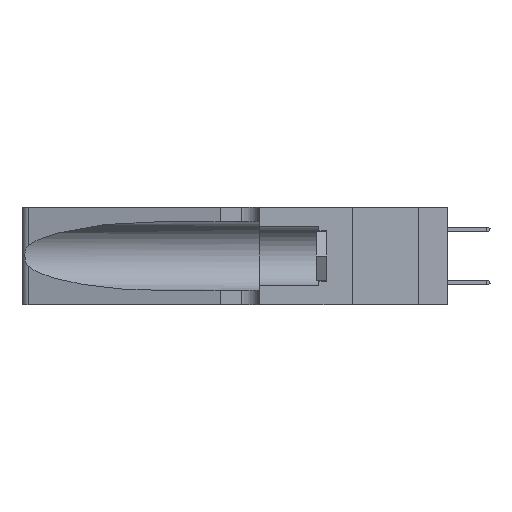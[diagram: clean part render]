
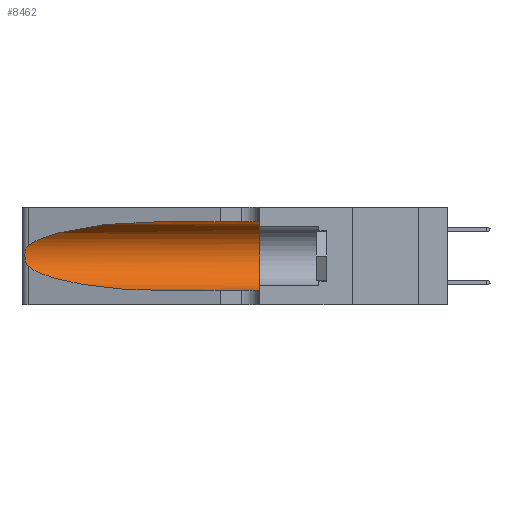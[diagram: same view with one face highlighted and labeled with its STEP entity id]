
A CAD part, left-side view. The second image highlights one B-rep face of the part: STEP entity #8462.
In plain terms, the highlighted cylindrical face has radius 3.308 mm (diameter 6.617 mm), a partial arc.
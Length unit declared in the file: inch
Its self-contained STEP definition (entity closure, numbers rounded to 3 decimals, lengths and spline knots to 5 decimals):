
#17 = EDGE_CURVE ( 'NONE', #8812, #5619, #6114, .T. ) ;
#32 = CARTESIAN_POINT ( 'NONE',  ( 0.25555, 1.22993, 0.14849 ) ) ;
#1219 = ORIENTED_EDGE ( 'NONE', *, *, #14206, .T. ) ;
#1509 = CARTESIAN_POINT ( 'NONE',  ( 0.25487, 1.22718, 0.22369 ) ) ;
#1870 = B_SPLINE_CURVE_WITH_KNOTS ( 'NONE', 3,
 ( #8646, #10775, #17141, #4388, #19278, #6592, #21378, #8741, #23460, #10874, #25539, #12975, #32, #15109 ),
 .UNSPECIFIED., .F., .F.,
 ( 4, 2, 2, 2, 2, 2, 4 ),
 ( 0., 0.00027, 0.00053, 0.00107, 0.0016, 0.00187, 0.00214 ),
 .UNSPECIFIED. ) ;
#2172 = FACE_OUTER_BOUND ( 'NONE', #9731, .T. ) ;
#3289 = VERTEX_POINT ( 'NONE', #6170 ) ;
#4388 = CARTESIAN_POINT ( 'NONE',  ( 0.25787, 1.23484, 0.2124 ) ) ;
#4996 = CARTESIAN_POINT ( 'NONE',  ( 0.25487, 1.22718, 0.14631 ) ) ;
#5226 = CARTESIAN_POINT ( 'NONE',  ( 0.1305, 0.72297, 0.05475 ) ) ;
#5433 = ORIENTED_EDGE ( 'NONE', *, *, #27164, .T. ) ;
#5501 = EDGE_CURVE ( 'NONE', #9207, #23455, #18853, .T. ) ;
#5619 = VERTEX_POINT ( 'NONE', #19487 ) ;
#5722 = AXIS2_PLACEMENT_3D ( 'NONE', #21940, #9316, #24040 ) ;
#5958 = VECTOR ( 'NONE', #11796, 39.37008 ) ;
#6114 =( BOUNDED_CURVE ( )  B_SPLINE_CURVE ( 3, ( #16597, #17229, #24713, #1509 ),
 .UNSPECIFIED., .F., .T. ) 
 B_SPLINE_CURVE_WITH_KNOTS ( ( 4, 4 ),
 ( 1.5708, 2.84003 ),
 .UNSPECIFIED. ) 
 CURVE ( )  GEOMETRIC_REPRESENTATION_ITEM ( )  RATIONAL_B_SPLINE_CURVE ( ( 1., 0.87, 0.87, 1. ) ) 
 REPRESENTATION_ITEM ( '' )  );
#6170 = CARTESIAN_POINT ( 'NONE',  ( 0.1305, 0.35, 0.31525 ) ) ;
#6348 = CARTESIAN_POINT ( 'NONE',  ( 0.25487, 1.22718, 0.14631 ) ) ;
#6394 = VECTOR ( 'NONE', #26778, 39.37008 ) ;
#6592 = CARTESIAN_POINT ( 'NONE',  ( 0.26018, 1.23835, 0.19895 ) ) ;
#6639 = CYLINDRICAL_SURFACE ( 'NONE', #16690, 0.13025 ) ;
#6921 = ORIENTED_EDGE ( 'NONE', *, *, #5501, .T. ) ;
#7614 = DIRECTION ( 'NONE',  ( 0., -1., 0. ) ) ;
#7970 = LINE ( 'NONE', #9660, #5958 ) ;
#8048 = ORIENTED_EDGE ( 'NONE', *, *, #17980, .F. ) ;
#8462 = ADVANCED_FACE ( 'NONE', ( #2172 ), #6639, .F. ) ;
#8500 = CARTESIAN_POINT ( 'NONE',  ( 0.1305, 0.72297, 0.05475 ) ) ;
#8646 = CARTESIAN_POINT ( 'NONE',  ( 0.25487, 1.22718, 0.22369 ) ) ;
#8741 = CARTESIAN_POINT ( 'NONE',  ( 0.26075, 1.23896, 0.178 ) ) ;
#8812 = VERTEX_POINT ( 'NONE', #26866 ) ;
#9207 = VERTEX_POINT ( 'NONE', #4996 ) ;
#9316 = DIRECTION ( 'NONE',  ( 0., 1., 0. ) ) ;
#9354 = CARTESIAN_POINT ( 'NONE',  ( 0.1305, 0.35, 0.05475 ) ) ;
#9660 = CARTESIAN_POINT ( 'NONE',  ( 0.1305, 1.61858, 0.05475 ) ) ;
#9731 = EDGE_LOOP ( 'NONE', ( #12218, #5433, #6921, #1219, #25384, #8048 ) ) ;
#10504 = VERTEX_POINT ( 'NONE', #9354 ) ;
#10775 = CARTESIAN_POINT ( 'NONE',  ( 0.25555, 1.22994, 0.2215 ) ) ;
#10874 = CARTESIAN_POINT ( 'NONE',  ( 0.25856, 1.23593, 0.16098 ) ) ;
#11130 = EDGE_CURVE ( 'NONE', #3289, #10504, #13754, .T. ) ;
#11786 = DIRECTION ( 'NONE',  ( 0., 0., -1. ) ) ;
#11796 = DIRECTION ( 'NONE',  ( 0., -1., 0. ) ) ;
#12218 = ORIENTED_EDGE ( 'NONE', *, *, #17, .T. ) ;
#12975 = CARTESIAN_POINT ( 'NONE',  ( 0.25639, 1.23186, 0.15144 ) ) ;
#13754 = CIRCLE ( 'NONE', #5722, 0.13025 ) ;
#14206 = EDGE_CURVE ( 'NONE', #23455, #10504, #7970, .T. ) ;
#15109 = CARTESIAN_POINT ( 'NONE',  ( 0.25487, 1.22718, 0.14631 ) ) ;
#16597 = CARTESIAN_POINT ( 'NONE',  ( 0.1305, 0.72297, 0.31525 ) ) ;
#16690 = AXIS2_PLACEMENT_3D ( 'NONE', #22353, #7614, #11786 ) ;
#16906 = CARTESIAN_POINT ( 'NONE',  ( 0.2373, 1.15595, 0.08982 ) ) ;
#17141 = CARTESIAN_POINT ( 'NONE',  ( 0.25639, 1.23184, 0.21858 ) ) ;
#17229 = CARTESIAN_POINT ( 'NONE',  ( 0.18966, 0.96281, 0.31525 ) ) ;
#17980 = EDGE_CURVE ( 'NONE', #8812, #3289, #23224, .T. ) ;
#18853 =( BOUNDED_CURVE ( )  B_SPLINE_CURVE ( 3, ( #6348, #16906, #21138, #8500 ),
 .UNSPECIFIED., .F., .F. ) 
 B_SPLINE_CURVE_WITH_KNOTS ( ( 4, 4 ),
 ( 3.44316, 4.71239 ),
 .UNSPECIFIED. ) 
 CURVE ( )  GEOMETRIC_REPRESENTATION_ITEM ( )  RATIONAL_B_SPLINE_CURVE ( ( 1., 0.87, 0.87, 1. ) ) 
 REPRESENTATION_ITEM ( '' )  );
#19278 = CARTESIAN_POINT ( 'NONE',  ( 0.25854, 1.2359, 0.20912 ) ) ;
#19487 = CARTESIAN_POINT ( 'NONE',  ( 0.25487, 1.22718, 0.22369 ) ) ;
#20513 = CARTESIAN_POINT ( 'NONE',  ( 0.1305, 1.61858, 0.31525 ) ) ;
#21138 = CARTESIAN_POINT ( 'NONE',  ( 0.18966, 0.96281, 0.05475 ) ) ;
#21378 = CARTESIAN_POINT ( 'NONE',  ( 0.26075, 1.23896, 0.19203 ) ) ;
#21940 = CARTESIAN_POINT ( 'NONE',  ( 0.1305, 0.35, 0.185 ) ) ;
#22353 = CARTESIAN_POINT ( 'NONE',  ( 0.1305, 1.61858, 0.185 ) ) ;
#23224 = LINE ( 'NONE', #20513, #6394 ) ;
#23455 = VERTEX_POINT ( 'NONE', #5226 ) ;
#23460 = CARTESIAN_POINT ( 'NONE',  ( 0.26017, 1.23833, 0.17102 ) ) ;
#24040 = DIRECTION ( 'NONE',  ( 0., 0., 1. ) ) ;
#24713 = CARTESIAN_POINT ( 'NONE',  ( 0.2373, 1.15595, 0.28018 ) ) ;
#25384 = ORIENTED_EDGE ( 'NONE', *, *, #11130, .F. ) ;
#25539 = CARTESIAN_POINT ( 'NONE',  ( 0.25789, 1.23486, 0.15765 ) ) ;
#26778 = DIRECTION ( 'NONE',  ( 0., -1., 0. ) ) ;
#26866 = CARTESIAN_POINT ( 'NONE',  ( 0.1305, 0.72297, 0.31525 ) ) ;
#27164 = EDGE_CURVE ( 'NONE', #5619, #9207, #1870, .T. ) ;
